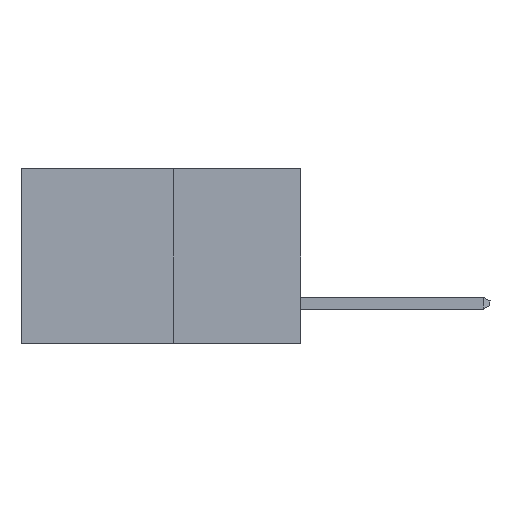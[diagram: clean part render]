
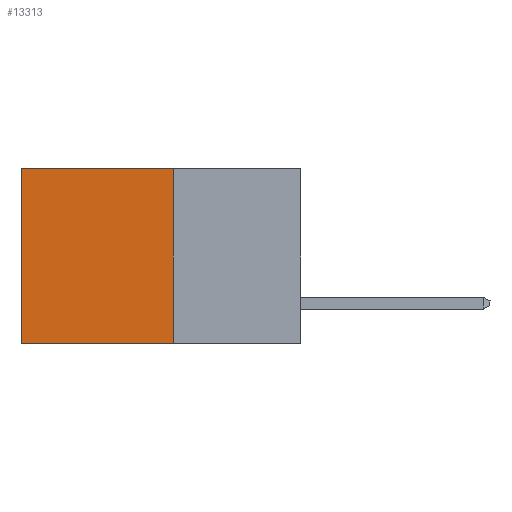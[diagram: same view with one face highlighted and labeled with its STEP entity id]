
A CAD part, left-side view. The second image highlights one B-rep face of the part: STEP entity #13313.
In plain terms, the highlighted planar face has unit normal (-1, 0, 0).
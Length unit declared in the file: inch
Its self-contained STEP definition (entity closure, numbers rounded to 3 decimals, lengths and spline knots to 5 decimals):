
#694 = PLANE ( 'NONE',  #8848 ) ;
#848 = DIRECTION ( 'NONE',  ( 0., 0., -1. ) ) ;
#943 = EDGE_CURVE ( 'NONE', #4113, #6237, #4260, .T. ) ;
#1122 = EDGE_CURVE ( 'NONE', #1167, #4113, #13491, .T. ) ;
#1167 = VERTEX_POINT ( 'NONE', #12806 ) ;
#1211 = CARTESIAN_POINT ( 'NONE',  ( 0.277, 0.59, -0.37 ) ) ;
#1297 = DIRECTION ( 'NONE',  ( 0., 0., -1. ) ) ;
#1349 = FACE_OUTER_BOUND ( 'NONE', #13312, .T. ) ;
#1579 = ORIENTED_EDGE ( 'NONE', *, *, #1122, .F. ) ;
#2375 = CARTESIAN_POINT ( 'NONE',  ( 0.277, 0.59, -0.37 ) ) ;
#2821 = CARTESIAN_POINT ( 'NONE',  ( 0.277, 0.27, -0.37 ) ) ;
#2841 = EDGE_CURVE ( 'NONE', #1167, #4445, #10014, .T. ) ;
#3577 = CARTESIAN_POINT ( 'NONE',  ( 0.277, 0.27, 0. ) ) ;
#3787 = EDGE_CURVE ( 'NONE', #4445, #6237, #12222, .T. ) ;
#4113 = VERTEX_POINT ( 'NONE', #4703 ) ;
#4260 = LINE ( 'NONE', #7947, #9703 ) ;
#4343 = DIRECTION ( 'NONE',  ( 1., 0., 0. ) ) ;
#4445 = VERTEX_POINT ( 'NONE', #10913 ) ;
#4703 = CARTESIAN_POINT ( 'NONE',  ( 0.277, 0.27, -0.37 ) ) ;
#5548 = DIRECTION ( 'NONE',  ( 0., 1., 0. ) ) ;
#6217 = ORIENTED_EDGE ( 'NONE', *, *, #943, .F. ) ;
#6237 = VERTEX_POINT ( 'NONE', #2375 ) ;
#6360 = VECTOR ( 'NONE', #848, 39.37008 ) ;
#7577 = ORIENTED_EDGE ( 'NONE', *, *, #2841, .T. ) ;
#7639 = VECTOR ( 'NONE', #1297, 39.37008 ) ;
#7947 = CARTESIAN_POINT ( 'NONE',  ( 0.277, 0.27, -0.37 ) ) ;
#8848 = AXIS2_PLACEMENT_3D ( 'NONE', #10886, #4343, #11992 ) ;
#9703 = VECTOR ( 'NONE', #13775, 39.37008 ) ;
#10014 = LINE ( 'NONE', #3577, #12252 ) ;
#10353 = ORIENTED_EDGE ( 'NONE', *, *, #3787, .T. ) ;
#10886 = CARTESIAN_POINT ( 'NONE',  ( 0.277, 0.27, -0.37 ) ) ;
#10913 = CARTESIAN_POINT ( 'NONE',  ( 0.277, 0.59, 0. ) ) ;
#11992 = DIRECTION ( 'NONE',  ( 0., 0., -1. ) ) ;
#12222 = LINE ( 'NONE', #1211, #6360 ) ;
#12252 = VECTOR ( 'NONE', #5548, 39.37008 ) ;
#12806 = CARTESIAN_POINT ( 'NONE',  ( 0.277, 0.27, 0. ) ) ;
#13312 = EDGE_LOOP ( 'NONE', ( #10353, #6217, #1579, #7577 ) ) ;
#13313 = ADVANCED_FACE ( 'NONE', ( #1349 ), #694, .F. ) ;
#13491 = LINE ( 'NONE', #2821, #7639 ) ;
#13775 = DIRECTION ( 'NONE',  ( 0., 1., 0. ) ) ;
